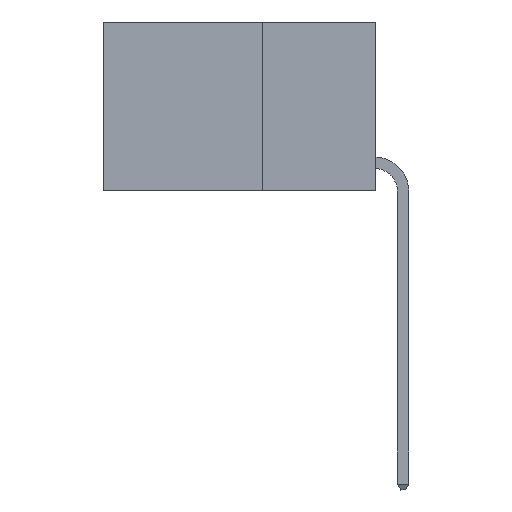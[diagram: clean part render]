
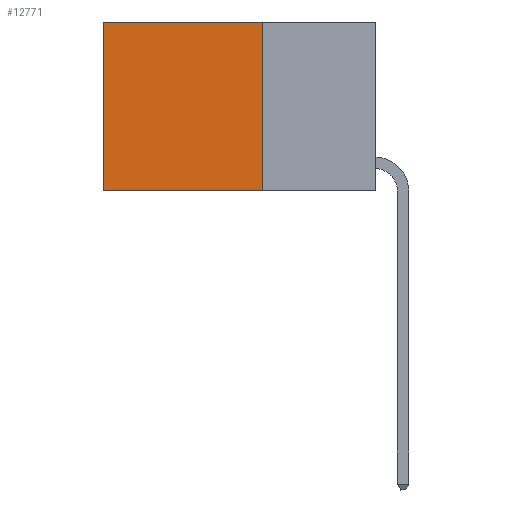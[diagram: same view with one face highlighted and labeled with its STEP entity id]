
A CAD part, left-side view. The second image highlights one B-rep face of the part: STEP entity #12771.
In plain terms, the highlighted planar face has unit normal (-1, 0, 0).
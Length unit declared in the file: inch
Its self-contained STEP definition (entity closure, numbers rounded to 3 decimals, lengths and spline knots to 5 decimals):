
#596 = VERTEX_POINT ( 'NONE', #13840 ) ;
#1506 = CARTESIAN_POINT ( 'NONE',  ( 0.2625, 0.25, -0.37 ) ) ;
#1672 = ORIENTED_EDGE ( 'NONE', *, *, #6144, .F. ) ;
#1718 = AXIS2_PLACEMENT_3D ( 'NONE', #5437, #6937, #17388 ) ;
#2097 = DIRECTION ( 'NONE',  ( 0., 1., 0. ) ) ;
#3629 = CARTESIAN_POINT ( 'NONE',  ( 0.2625, 0.25, 0. ) ) ;
#3778 = VERTEX_POINT ( 'NONE', #8988 ) ;
#4042 = EDGE_CURVE ( 'NONE', #3778, #596, #15542, .T. ) ;
#5437 = CARTESIAN_POINT ( 'NONE',  ( 0.2625, 0.25, 0. ) ) ;
#6021 = CARTESIAN_POINT ( 'NONE',  ( 0.2625, 0.25, -0.37 ) ) ;
#6144 = EDGE_CURVE ( 'NONE', #3778, #18072, #7769, .T. ) ;
#6937 = DIRECTION ( 'NONE',  ( 1., 0., 0. ) ) ;
#7482 = LINE ( 'NONE', #16075, #18424 ) ;
#7627 = CARTESIAN_POINT ( 'NONE',  ( 0.2625, 0.25, 0. ) ) ;
#7703 = EDGE_CURVE ( 'NONE', #596, #11787, #7482, .T. ) ;
#7769 = LINE ( 'NONE', #7627, #19184 ) ;
#8072 = VECTOR ( 'NONE', #2097, 39.37008 ) ;
#8640 = DIRECTION ( 'NONE',  ( 0., 0., -1. ) ) ;
#8988 = CARTESIAN_POINT ( 'NONE',  ( 0.2625, 0.25, 0. ) ) ;
#10643 = EDGE_LOOP ( 'NONE', ( #15758, #14456, #1672, #14438 ) ) ;
#11787 = VERTEX_POINT ( 'NONE', #14683 ) ;
#12771 = ADVANCED_FACE ( 'NONE', ( #19055 ), #14117, .F. ) ;
#13631 = DIRECTION ( 'NONE',  ( 0., 0., -1. ) ) ;
#13840 = CARTESIAN_POINT ( 'NONE',  ( 0.2625, 0.6, 0. ) ) ;
#14117 = PLANE ( 'NONE',  #1718 ) ;
#14438 = ORIENTED_EDGE ( 'NONE', *, *, #4042, .T. ) ;
#14456 = ORIENTED_EDGE ( 'NONE', *, *, #16405, .F. ) ;
#14683 = CARTESIAN_POINT ( 'NONE',  ( 0.2625, 0.6, -0.37 ) ) ;
#15344 = VECTOR ( 'NONE', #19365, 39.37008 ) ;
#15542 = LINE ( 'NONE', #3629, #8072 ) ;
#15758 = ORIENTED_EDGE ( 'NONE', *, *, #7703, .T. ) ;
#15812 = LINE ( 'NONE', #1506, #15344 ) ;
#16075 = CARTESIAN_POINT ( 'NONE',  ( 0.2625, 0.6, 0. ) ) ;
#16405 = EDGE_CURVE ( 'NONE', #18072, #11787, #15812, .T. ) ;
#17388 = DIRECTION ( 'NONE',  ( 0., 0., -1. ) ) ;
#18072 = VERTEX_POINT ( 'NONE', #6021 ) ;
#18424 = VECTOR ( 'NONE', #8640, 39.37008 ) ;
#19055 = FACE_OUTER_BOUND ( 'NONE', #10643, .T. ) ;
#19184 = VECTOR ( 'NONE', #13631, 39.37008 ) ;
#19365 = DIRECTION ( 'NONE',  ( 0., 1., 0. ) ) ;
